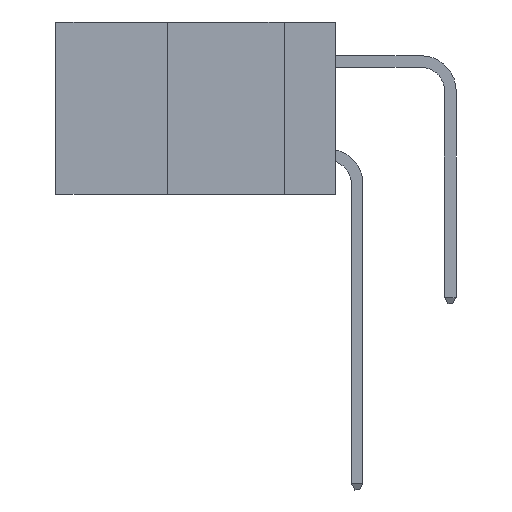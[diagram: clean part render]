
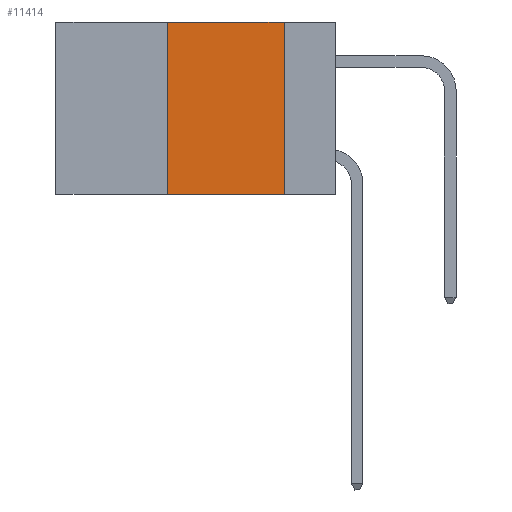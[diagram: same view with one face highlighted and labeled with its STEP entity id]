
A CAD part, left-side view. The second image highlights one B-rep face of the part: STEP entity #11414.
In plain terms, the highlighted planar face has unit normal (-1, 0, 0).
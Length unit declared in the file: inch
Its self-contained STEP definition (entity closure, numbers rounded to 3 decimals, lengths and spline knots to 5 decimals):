
#1251 = CARTESIAN_POINT ( 'NONE',  ( 0., 0.11, -0.37 ) ) ;
#1800 = VECTOR ( 'NONE', #24617, 39.37008 ) ;
#2446 = VERTEX_POINT ( 'NONE', #1251 ) ;
#2623 = VECTOR ( 'NONE', #4117, 39.37008 ) ;
#2700 = CARTESIAN_POINT ( 'NONE',  ( 0., 0.36, -0.37 ) ) ;
#3832 = DIRECTION ( 'NONE',  ( 1., 0., 0. ) ) ;
#4117 = DIRECTION ( 'NONE',  ( 0., 0., 1. ) ) ;
#4587 = CARTESIAN_POINT ( 'NONE',  ( 0., 0.36, 0. ) ) ;
#6138 = LINE ( 'NONE', #11370, #15981 ) ;
#6953 = VECTOR ( 'NONE', #13418, 39.37008 ) ;
#7252 = LINE ( 'NONE', #22668, #1800 ) ;
#8067 = EDGE_CURVE ( 'NONE', #18698, #25490, #13278, .T. ) ;
#8608 = EDGE_CURVE ( 'NONE', #25490, #12614, #6138, .T. ) ;
#11195 = EDGE_CURVE ( 'NONE', #12614, #2446, #7252, .T. ) ;
#11370 = CARTESIAN_POINT ( 'NONE',  ( 0., 0.6, 0. ) ) ;
#11414 = ADVANCED_FACE ( 'NONE', ( #12136 ), #25266, .F. ) ;
#11541 = LINE ( 'NONE', #19266, #6953 ) ;
#12136 = FACE_OUTER_BOUND ( 'NONE', #19140, .T. ) ;
#12236 = AXIS2_PLACEMENT_3D ( 'NONE', #15709, #3832, #17643 ) ;
#12614 = VERTEX_POINT ( 'NONE', #17279 ) ;
#13278 = LINE ( 'NONE', #19866, #2623 ) ;
#13418 = DIRECTION ( 'NONE',  ( 0., -1., 0. ) ) ;
#14068 = ORIENTED_EDGE ( 'NONE', *, *, #11195, .F. ) ;
#15709 = CARTESIAN_POINT ( 'NONE',  ( 0., 0.6, 0. ) ) ;
#15981 = VECTOR ( 'NONE', #22955, 39.37008 ) ;
#17279 = CARTESIAN_POINT ( 'NONE',  ( 0., 0.11, 0. ) ) ;
#17643 = DIRECTION ( 'NONE',  ( 0., 0., -1. ) ) ;
#17728 = EDGE_CURVE ( 'NONE', #18698, #2446, #11541, .T. ) ;
#18698 = VERTEX_POINT ( 'NONE', #2700 ) ;
#19140 = EDGE_LOOP ( 'NONE', ( #14068, #19224, #20418, #22801 ) ) ;
#19224 = ORIENTED_EDGE ( 'NONE', *, *, #8608, .F. ) ;
#19266 = CARTESIAN_POINT ( 'NONE',  ( 0., 0.6, -0.37 ) ) ;
#19866 = CARTESIAN_POINT ( 'NONE',  ( 0., 0.36, 0. ) ) ;
#20418 = ORIENTED_EDGE ( 'NONE', *, *, #8067, .F. ) ;
#22668 = CARTESIAN_POINT ( 'NONE',  ( 0., 0.11, 0. ) ) ;
#22801 = ORIENTED_EDGE ( 'NONE', *, *, #17728, .T. ) ;
#22955 = DIRECTION ( 'NONE',  ( 0., -1., 0. ) ) ;
#24617 = DIRECTION ( 'NONE',  ( 0., 0., -1. ) ) ;
#25266 = PLANE ( 'NONE',  #12236 ) ;
#25490 = VERTEX_POINT ( 'NONE', #4587 ) ;
